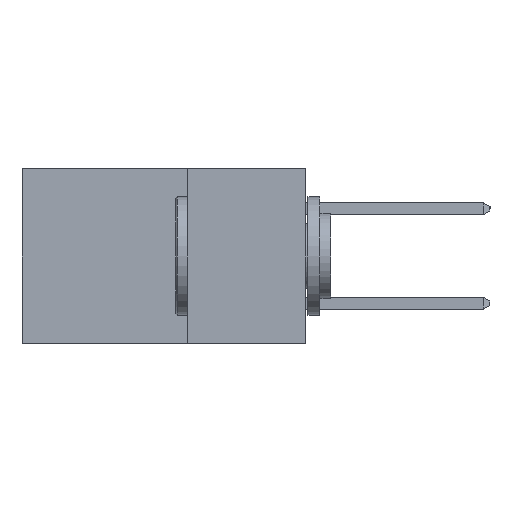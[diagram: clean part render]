
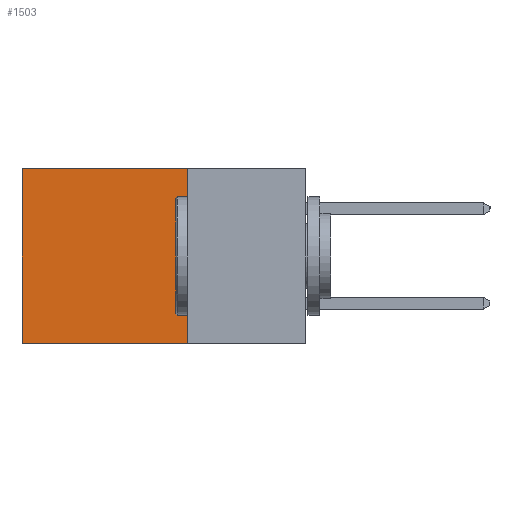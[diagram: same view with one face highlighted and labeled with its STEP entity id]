
A CAD part, left-side view. The second image highlights one B-rep face of the part: STEP entity #1503.
In plain terms, the highlighted planar face has unit normal (-1, 0, 0).
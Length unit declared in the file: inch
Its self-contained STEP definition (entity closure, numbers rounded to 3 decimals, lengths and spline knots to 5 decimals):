
#101 = DIRECTION ( 'NONE',  ( 0., 0., -1. ) ) ;
#1428 = VECTOR ( 'NONE', #10231, 39.37008 ) ;
#1503 = ADVANCED_FACE ( 'NONE', ( #14238 ), #13870, .F. ) ;
#1951 = VERTEX_POINT ( 'NONE', #11633 ) ;
#2317 = VECTOR ( 'NONE', #17491, 39.37008 ) ;
#4508 = ORIENTED_EDGE ( 'NONE', *, *, #18856, .F. ) ;
#4893 = CARTESIAN_POINT ( 'NONE',  ( 0.2615, 0.25, -0.37 ) ) ;
#6361 = EDGE_CURVE ( 'NONE', #13765, #1951, #19982, .T. ) ;
#6729 = CARTESIAN_POINT ( 'NONE',  ( 0.2615, 0.25, -0.37 ) ) ;
#8428 = EDGE_CURVE ( 'NONE', #9247, #13765, #21741, .T. ) ;
#8662 = LINE ( 'NONE', #6729, #1428 ) ;
#9059 = ORIENTED_EDGE ( 'NONE', *, *, #20287, .F. ) ;
#9247 = VERTEX_POINT ( 'NONE', #16390 ) ;
#9673 = CARTESIAN_POINT ( 'NONE',  ( 0.2615, 0.25, 0. ) ) ;
#9818 = EDGE_LOOP ( 'NONE', ( #21641, #9059, #4508, #15790 ) ) ;
#10231 = DIRECTION ( 'NONE',  ( 0., 0., -1. ) ) ;
#11633 = CARTESIAN_POINT ( 'NONE',  ( 0.2615, 0.6, -0.37 ) ) ;
#11914 = CARTESIAN_POINT ( 'NONE',  ( 0.2615, 0.25, -0.37 ) ) ;
#13756 = VECTOR ( 'NONE', #25277, 39.37008 ) ;
#13765 = VERTEX_POINT ( 'NONE', #24569 ) ;
#13870 = PLANE ( 'NONE',  #18114 ) ;
#14046 = VERTEX_POINT ( 'NONE', #4893 ) ;
#14238 = FACE_OUTER_BOUND ( 'NONE', #9818, .T. ) ;
#15757 = VECTOR ( 'NONE', #24027, 39.37008 ) ;
#15790 = ORIENTED_EDGE ( 'NONE', *, *, #8428, .T. ) ;
#16390 = CARTESIAN_POINT ( 'NONE',  ( 0.2615, 0.25, 0. ) ) ;
#17491 = DIRECTION ( 'NONE',  ( 0., 1., 0. ) ) ;
#18114 = AXIS2_PLACEMENT_3D ( 'NONE', #11914, #19841, #101 ) ;
#18856 = EDGE_CURVE ( 'NONE', #9247, #14046, #8662, .T. ) ;
#19841 = DIRECTION ( 'NONE',  ( 1., 0., 0. ) ) ;
#19982 = LINE ( 'NONE', #22060, #15757 ) ;
#20287 = EDGE_CURVE ( 'NONE', #14046, #1951, #25319, .T. ) ;
#21641 = ORIENTED_EDGE ( 'NONE', *, *, #6361, .T. ) ;
#21741 = LINE ( 'NONE', #9673, #13756 ) ;
#22060 = CARTESIAN_POINT ( 'NONE',  ( 0.2615, 0.6, -0.37 ) ) ;
#23359 = CARTESIAN_POINT ( 'NONE',  ( 0.2615, 0.25, -0.37 ) ) ;
#24027 = DIRECTION ( 'NONE',  ( 0., 0., -1. ) ) ;
#24569 = CARTESIAN_POINT ( 'NONE',  ( 0.2615, 0.6, 0. ) ) ;
#25277 = DIRECTION ( 'NONE',  ( 0., 1., 0. ) ) ;
#25319 = LINE ( 'NONE', #23359, #2317 ) ;
